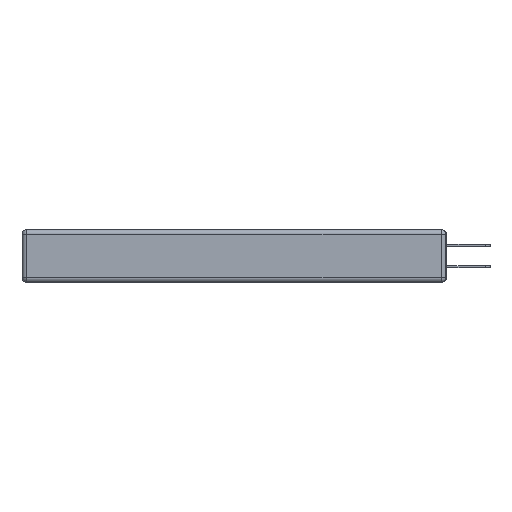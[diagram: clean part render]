
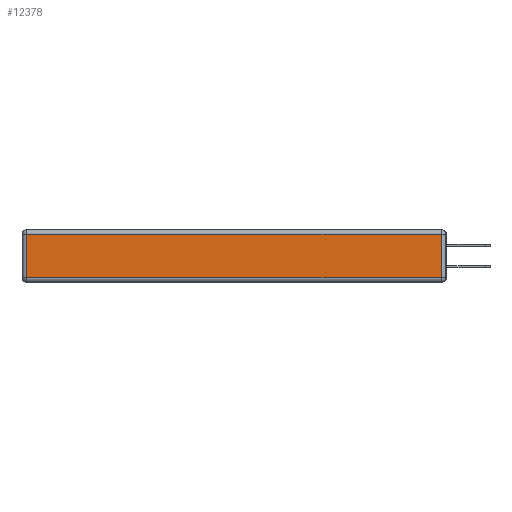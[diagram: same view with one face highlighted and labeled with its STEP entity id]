
A CAD part, left-side view. The second image highlights one B-rep face of the part: STEP entity #12378.
In plain terms, the highlighted planar face has unit normal (-1, 0, 0).
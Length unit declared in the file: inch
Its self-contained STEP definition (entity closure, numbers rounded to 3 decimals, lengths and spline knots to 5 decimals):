
#13 = ORIENTED_EDGE ( 'NONE', *, *, #14413, .T. ) ;
#856 = DIRECTION ( 'NONE',  ( 0., 0., -1. ) ) ;
#1546 = AXIS2_PLACEMENT_3D ( 'NONE', #15359, #16970, #2875 ) ;
#1720 = ORIENTED_EDGE ( 'NONE', *, *, #10746, .T. ) ;
#1785 = ORIENTED_EDGE ( 'NONE', *, *, #6657, .T. ) ;
#2680 = VECTOR ( 'NONE', #14274, 39.37008 ) ;
#2875 = DIRECTION ( 'NONE',  ( 0., 0., 1. ) ) ;
#3117 = LINE ( 'NONE', #18798, #16396 ) ;
#3142 = VECTOR ( 'NONE', #856, 39.37008 ) ;
#4253 = VERTEX_POINT ( 'NONE', #14350 ) ;
#4373 = PLANE ( 'NONE',  #1546 ) ;
#4640 = LINE ( 'NONE', #4786, #2680 ) ;
#4786 = CARTESIAN_POINT ( 'NONE',  ( 0., 0.03, -0.343 ) ) ;
#4821 = DIRECTION ( 'NONE',  ( 0., 1., 0. ) ) ;
#6070 = CARTESIAN_POINT ( 'NONE',  ( 0., 2.72, -0.03 ) ) ;
#6657 = EDGE_CURVE ( 'NONE', #4253, #17576, #3117, .T. ) ;
#7312 = CARTESIAN_POINT ( 'NONE',  ( 0., 2.72, -0.343 ) ) ;
#7670 = LINE ( 'NONE', #16028, #13070 ) ;
#9153 = VERTEX_POINT ( 'NONE', #6070 ) ;
#9770 = ORIENTED_EDGE ( 'NONE', *, *, #10366, .T. ) ;
#10366 = EDGE_CURVE ( 'NONE', #17576, #18292, #4640, .T. ) ;
#10746 = EDGE_CURVE ( 'NONE', #9153, #4253, #18659, .T. ) ;
#12378 = ADVANCED_FACE ( 'NONE', ( #15357 ), #4373, .T. ) ;
#13070 = VECTOR ( 'NONE', #4821, 39.37008 ) ;
#14079 = EDGE_LOOP ( 'NONE', ( #1785, #9770, #13, #1720 ) ) ;
#14274 = DIRECTION ( 'NONE',  ( 0., 0., 1. ) ) ;
#14298 = DIRECTION ( 'NONE',  ( 0., -1., 0. ) ) ;
#14311 = CARTESIAN_POINT ( 'NONE',  ( 0., 0.03, -0.313 ) ) ;
#14350 = CARTESIAN_POINT ( 'NONE',  ( 0., 2.72, -0.313 ) ) ;
#14413 = EDGE_CURVE ( 'NONE', #18292, #9153, #7670, .T. ) ;
#15357 = FACE_OUTER_BOUND ( 'NONE', #14079, .T. ) ;
#15359 = CARTESIAN_POINT ( 'NONE',  ( 0., 0., -0.343 ) ) ;
#16028 = CARTESIAN_POINT ( 'NONE',  ( 0., 2.75, -0.03 ) ) ;
#16396 = VECTOR ( 'NONE', #14298, 39.37008 ) ;
#16899 = CARTESIAN_POINT ( 'NONE',  ( 0., 0.03, -0.03 ) ) ;
#16970 = DIRECTION ( 'NONE',  ( -1., 0., 0. ) ) ;
#17576 = VERTEX_POINT ( 'NONE', #14311 ) ;
#18292 = VERTEX_POINT ( 'NONE', #16899 ) ;
#18659 = LINE ( 'NONE', #7312, #3142 ) ;
#18798 = CARTESIAN_POINT ( 'NONE',  ( 0., 0., -0.313 ) ) ;
